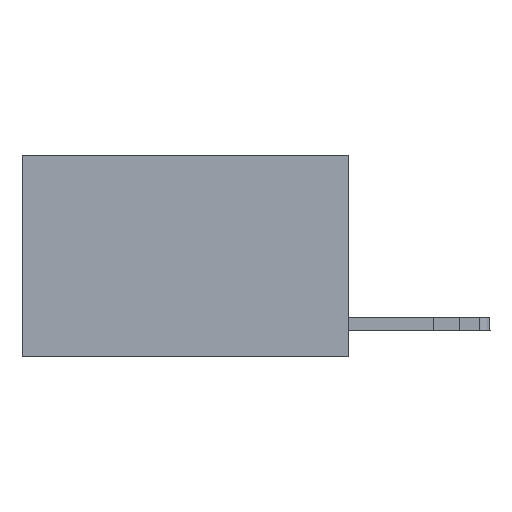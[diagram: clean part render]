
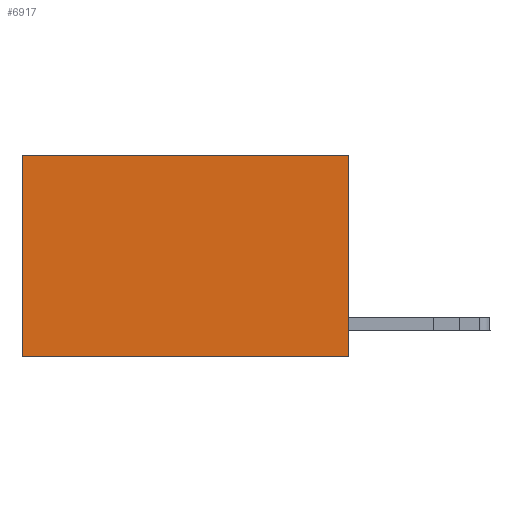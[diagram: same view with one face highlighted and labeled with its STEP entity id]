
A CAD part, left-side view. The second image highlights one B-rep face of the part: STEP entity #6917.
In plain terms, the highlighted planar face has unit normal (-1, 0, 0).
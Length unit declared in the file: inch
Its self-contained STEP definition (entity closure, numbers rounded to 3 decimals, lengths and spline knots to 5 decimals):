
#251 = VECTOR ( 'NONE', #6224, 39.37008 ) ;
#443 = CARTESIAN_POINT ( 'NONE',  ( 0.2625, 0.6, -0.37 ) ) ;
#932 = VECTOR ( 'NONE', #3712, 39.37008 ) ;
#1427 = VERTEX_POINT ( 'NONE', #21207 ) ;
#3097 = ORIENTED_EDGE ( 'NONE', *, *, #3906, .T. ) ;
#3712 = DIRECTION ( 'NONE',  ( 0., 0., -1. ) ) ;
#3906 = EDGE_CURVE ( 'NONE', #16162, #13645, #17341, .T. ) ;
#4536 = EDGE_CURVE ( 'NONE', #23443, #16162, #15624, .T. ) ;
#4671 = VECTOR ( 'NONE', #23166, 39.37008 ) ;
#6224 = DIRECTION ( 'NONE',  ( 0., 0., -1. ) ) ;
#6771 = ORIENTED_EDGE ( 'NONE', *, *, #4536, .T. ) ;
#6917 = ADVANCED_FACE ( 'NONE', ( #16390 ), #6989, .F. ) ;
#6989 = PLANE ( 'NONE',  #9330 ) ;
#7872 = DIRECTION ( 'NONE',  ( 0., 1., 0. ) ) ;
#9330 = AXIS2_PLACEMENT_3D ( 'NONE', #12448, #12566, #19640 ) ;
#9745 = CARTESIAN_POINT ( 'NONE',  ( 0.2625, 0.6, 0. ) ) ;
#10753 = CARTESIAN_POINT ( 'NONE',  ( 0.2625, 0.6, 0. ) ) ;
#11352 = LINE ( 'NONE', #13138, #932 ) ;
#11772 = CARTESIAN_POINT ( 'NONE',  ( 0.2625, 0., -0.37 ) ) ;
#12448 = CARTESIAN_POINT ( 'NONE',  ( 0.2625, 0., 0. ) ) ;
#12566 = DIRECTION ( 'NONE',  ( 1., 0., 0. ) ) ;
#13138 = CARTESIAN_POINT ( 'NONE',  ( 0.2625, 0., 0. ) ) ;
#13537 = LINE ( 'NONE', #11772, #15537 ) ;
#13645 = VERTEX_POINT ( 'NONE', #443 ) ;
#13681 = EDGE_LOOP ( 'NONE', ( #3097, #16361, #17392, #6771 ) ) ;
#15537 = VECTOR ( 'NONE', #7872, 39.37008 ) ;
#15624 = LINE ( 'NONE', #21626, #4671 ) ;
#16162 = VERTEX_POINT ( 'NONE', #10753 ) ;
#16271 = EDGE_CURVE ( 'NONE', #23443, #1427, #11352, .T. ) ;
#16361 = ORIENTED_EDGE ( 'NONE', *, *, #18659, .F. ) ;
#16390 = FACE_OUTER_BOUND ( 'NONE', #13681, .T. ) ;
#17341 = LINE ( 'NONE', #9745, #251 ) ;
#17392 = ORIENTED_EDGE ( 'NONE', *, *, #16271, .F. ) ;
#18659 = EDGE_CURVE ( 'NONE', #1427, #13645, #13537, .T. ) ;
#19640 = DIRECTION ( 'NONE',  ( 0., 0., -1. ) ) ;
#21207 = CARTESIAN_POINT ( 'NONE',  ( 0.2625, 0., -0.37 ) ) ;
#21626 = CARTESIAN_POINT ( 'NONE',  ( 0.2625, 0., 0. ) ) ;
#21913 = CARTESIAN_POINT ( 'NONE',  ( 0.2625, 0., 0. ) ) ;
#23166 = DIRECTION ( 'NONE',  ( 0., 1., 0. ) ) ;
#23443 = VERTEX_POINT ( 'NONE', #21913 ) ;
